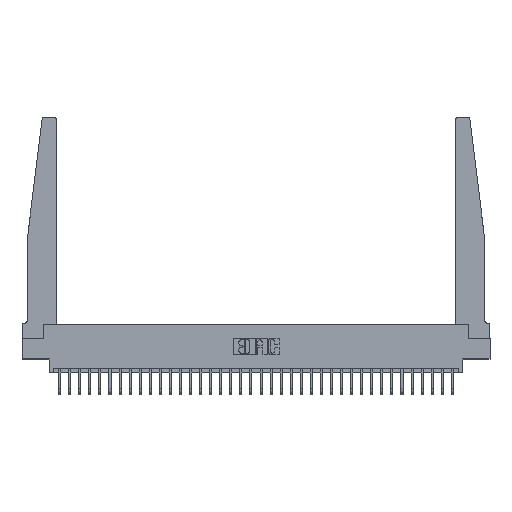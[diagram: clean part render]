
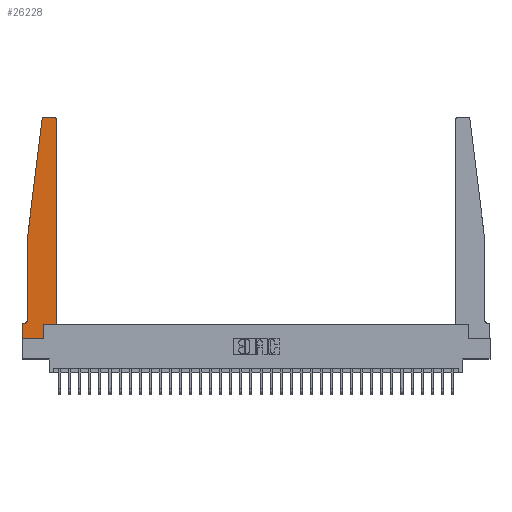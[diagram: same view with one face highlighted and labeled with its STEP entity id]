
A CAD part, top view. The second image highlights one B-rep face of the part: STEP entity #26228.
In plain terms, the highlighted planar face has unit normal (0, 0, 1).
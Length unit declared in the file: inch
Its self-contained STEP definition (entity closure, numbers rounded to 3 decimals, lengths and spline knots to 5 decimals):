
#63 = DIRECTION ( 'NONE',  ( -1., 0., 0. ) ) ;
#457 = LINE ( 'NONE', #4631, #19093 ) ;
#1133 = LINE ( 'NONE', #1502, #12944 ) ;
#1187 = DIRECTION ( 'NONE',  ( 0., 0., 1. ) ) ;
#1395 = VERTEX_POINT ( 'NONE', #20100 ) ;
#1455 = VERTEX_POINT ( 'NONE', #27219 ) ;
#1502 = CARTESIAN_POINT ( 'NONE',  ( 0.425, 0.18, 0.37 ) ) ;
#2548 = LINE ( 'NONE', #5342, #15014 ) ;
#2661 = VERTEX_POINT ( 'NONE', #10618 ) ;
#3060 = CARTESIAN_POINT ( 'NONE',  ( 0.065, 1.25, 0.37 ) ) ;
#3337 = VERTEX_POINT ( 'NONE', #24506 ) ;
#3784 = CARTESIAN_POINT ( 'NONE',  ( 0.425, 0.18, 0.37 ) ) ;
#3874 = VERTEX_POINT ( 'NONE', #19841 ) ;
#4330 = DIRECTION ( 'NONE',  ( 0., -1., 0. ) ) ;
#4631 = CARTESIAN_POINT ( 'NONE',  ( 0.2605, 0.18, 0.37 ) ) ;
#4669 = ORIENTED_EDGE ( 'NONE', *, *, #21698, .T. ) ;
#5017 = LINE ( 'NONE', #21405, #21308 ) ;
#5096 = VECTOR ( 'NONE', #19804, 39.37008 ) ;
#5342 = CARTESIAN_POINT ( 'NONE',  ( 0.065, 1.25, 0.37 ) ) ;
#5362 = ORIENTED_EDGE ( 'NONE', *, *, #14429, .T. ) ;
#6300 = DIRECTION ( 'NONE',  ( 0., 1., 0. ) ) ;
#6309 = CARTESIAN_POINT ( 'NONE',  ( 0.425, 2.72, 0.37 ) ) ;
#6489 = ORIENTED_EDGE ( 'NONE', *, *, #24740, .T. ) ;
#7097 = DIRECTION ( 'NONE',  ( 1., 0., 0. ) ) ;
#7151 = CARTESIAN_POINT ( 'NONE',  ( 0.2605, 0., 0.37 ) ) ;
#7625 = ORIENTED_EDGE ( 'NONE', *, *, #24865, .T. ) ;
#7801 = DIRECTION ( 'NONE',  ( 0., 0., 1. ) ) ;
#8643 = EDGE_CURVE ( 'NONE', #1455, #14219, #2548, .T. ) ;
#8890 = CIRCLE ( 'NONE', #26057, 0.03 ) ;
#9167 = CIRCLE ( 'NONE', #14623, 0.05 ) ;
#9422 = ORIENTED_EDGE ( 'NONE', *, *, #15222, .T. ) ;
#9741 = AXIS2_PLACEMENT_3D ( 'NONE', #10032, #26156, #12398 ) ;
#9773 = EDGE_LOOP ( 'NONE', ( #20981, #7625, #12369, #17036, #23879, #9422, #4669, #6489, #21414, #5362, #16982, #10096 ) ) ;
#10032 = CARTESIAN_POINT ( 'NONE',  ( 0.27653, 2.72, 0.37 ) ) ;
#10096 = ORIENTED_EDGE ( 'NONE', *, *, #28457, .T. ) ;
#10261 = CARTESIAN_POINT ( 'NONE',  ( 0.015, 0.2375, 0.37 ) ) ;
#10618 = CARTESIAN_POINT ( 'NONE',  ( 0.27653, 2.75, 0.37 ) ) ;
#12357 = EDGE_CURVE ( 'NONE', #3337, #26976, #9167, .T. ) ;
#12369 = ORIENTED_EDGE ( 'NONE', *, *, #8643, .T. ) ;
#12398 = DIRECTION ( 'NONE',  ( 1., 0., 0. ) ) ;
#12629 = DIRECTION ( 'NONE',  ( -1., 0., 0. ) ) ;
#12944 = VECTOR ( 'NONE', #6300, 39.37008 ) ;
#13037 = CARTESIAN_POINT ( 'NONE',  ( 0., 0., 0.37 ) ) ;
#13194 = EDGE_CURVE ( 'NONE', #20545, #2661, #23556, .T. ) ;
#14127 = LINE ( 'NONE', #3784, #24917 ) ;
#14175 = CARTESIAN_POINT ( 'NONE',  ( 0.065, 0.1875, 0.37 ) ) ;
#14219 = VERTEX_POINT ( 'NONE', #3060 ) ;
#14429 = EDGE_CURVE ( 'NONE', #1395, #23943, #14127, .T. ) ;
#14584 = DIRECTION ( 'NONE',  ( 0., -1., 0. ) ) ;
#14610 = DIRECTION ( 'NONE',  ( -0.122, -0.992, 0. ) ) ;
#14623 = AXIS2_PLACEMENT_3D ( 'NONE', #10261, #26381, #12629 ) ;
#15014 = VECTOR ( 'NONE', #14610, 39.37008 ) ;
#15222 = EDGE_CURVE ( 'NONE', #26976, #3874, #29862, .T. ) ;
#15934 = CARTESIAN_POINT ( 'NONE',  ( 0., 0., 0.37 ) ) ;
#16982 = ORIENTED_EDGE ( 'NONE', *, *, #28088, .T. ) ;
#17036 = ORIENTED_EDGE ( 'NONE', *, *, #25531, .T. ) ;
#17444 = CARTESIAN_POINT ( 'NONE',  ( 0., 0.1875, 0.37 ) ) ;
#17547 = DIRECTION ( 'NONE',  ( 1., 0., 0. ) ) ;
#18489 = LINE ( 'NONE', #18625, #23888 ) ;
#18625 = CARTESIAN_POINT ( 'NONE',  ( 0., 0., 0.37 ) ) ;
#18700 = CARTESIAN_POINT ( 'NONE',  ( 0.015, 0.1875, 0.37 ) ) ;
#19093 = VECTOR ( 'NONE', #27674, 39.37008 ) ;
#19804 = DIRECTION ( 'NONE',  ( -1., 0., 0. ) ) ;
#19841 = CARTESIAN_POINT ( 'NONE',  ( 0., 0.1875, 0.37 ) ) ;
#20100 = CARTESIAN_POINT ( 'NONE',  ( 0.2605, 0.18, 0.37 ) ) ;
#20545 = VERTEX_POINT ( 'NONE', #21553 ) ;
#20981 = ORIENTED_EDGE ( 'NONE', *, *, #13194, .T. ) ;
#21308 = VECTOR ( 'NONE', #14584, 39.37008 ) ;
#21405 = CARTESIAN_POINT ( 'NONE',  ( 0.065, 1.25, 0.37 ) ) ;
#21414 = ORIENTED_EDGE ( 'NONE', *, *, #26562, .T. ) ;
#21553 = CARTESIAN_POINT ( 'NONE',  ( 0.395, 2.75, 0.37 ) ) ;
#21633 = CARTESIAN_POINT ( 'NONE',  ( 0.395, 2.72, 0.37 ) ) ;
#21698 = EDGE_CURVE ( 'NONE', #3874, #24533, #24128, .T. ) ;
#21727 = CIRCLE ( 'NONE', #9741, 0.03 ) ;
#22120 = CARTESIAN_POINT ( 'NONE',  ( 0.25, 2.75, 0.37 ) ) ;
#22368 = DIRECTION ( 'NONE',  ( 1., 0., 0. ) ) ;
#22564 = CARTESIAN_POINT ( 'NONE',  ( 0.425, 0.18, 0.37 ) ) ;
#22696 = VECTOR ( 'NONE', #4330, 39.37008 ) ;
#23072 = VECTOR ( 'NONE', #63, 39.37008 ) ;
#23556 = LINE ( 'NONE', #22120, #5096 ) ;
#23879 = ORIENTED_EDGE ( 'NONE', *, *, #12357, .T. ) ;
#23888 = VECTOR ( 'NONE', #7097, 39.37008 ) ;
#23943 = VERTEX_POINT ( 'NONE', #22564 ) ;
#23953 = DIRECTION ( 'NONE',  ( 1., 0., 0. ) ) ;
#24128 = LINE ( 'NONE', #15934, #22696 ) ;
#24473 = AXIS2_PLACEMENT_3D ( 'NONE', #17444, #1187, #17547 ) ;
#24506 = CARTESIAN_POINT ( 'NONE',  ( 0.065, 0.2375, 0.37 ) ) ;
#24533 = VERTEX_POINT ( 'NONE', #13037 ) ;
#24598 = VERTEX_POINT ( 'NONE', #6309 ) ;
#24740 = EDGE_CURVE ( 'NONE', #24533, #25942, #18489, .T. ) ;
#24865 = EDGE_CURVE ( 'NONE', #2661, #1455, #21727, .T. ) ;
#24917 = VECTOR ( 'NONE', #22368, 39.37008 ) ;
#25531 = EDGE_CURVE ( 'NONE', #14219, #3337, #5017, .T. ) ;
#25942 = VERTEX_POINT ( 'NONE', #7151 ) ;
#26057 = AXIS2_PLACEMENT_3D ( 'NONE', #21633, #7801, #23953 ) ;
#26156 = DIRECTION ( 'NONE',  ( 0., 0., 1. ) ) ;
#26228 = ADVANCED_FACE ( 'NONE', ( #27018 ), #28993, .T. ) ;
#26381 = DIRECTION ( 'NONE',  ( 0., 0., -1. ) ) ;
#26562 = EDGE_CURVE ( 'NONE', #25942, #1395, #457, .T. ) ;
#26976 = VERTEX_POINT ( 'NONE', #18700 ) ;
#27018 = FACE_OUTER_BOUND ( 'NONE', #9773, .T. ) ;
#27219 = CARTESIAN_POINT ( 'NONE',  ( 0.24675, 2.72367, 0.37 ) ) ;
#27674 = DIRECTION ( 'NONE',  ( 0., 1., 0. ) ) ;
#28088 = EDGE_CURVE ( 'NONE', #23943, #24598, #1133, .T. ) ;
#28457 = EDGE_CURVE ( 'NONE', #24598, #20545, #8890, .T. ) ;
#28993 = PLANE ( 'NONE',  #24473 ) ;
#29862 = LINE ( 'NONE', #14175, #23072 ) ;
